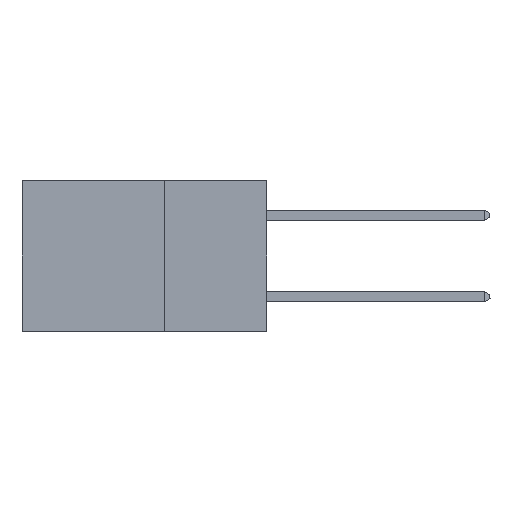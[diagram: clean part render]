
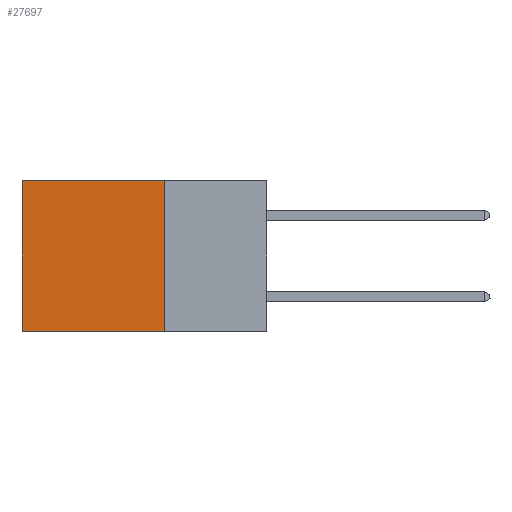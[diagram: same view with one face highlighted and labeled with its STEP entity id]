
A CAD part, left-side view. The second image highlights one B-rep face of the part: STEP entity #27697.
In plain terms, the highlighted planar face has unit normal (-1, 0, 0).
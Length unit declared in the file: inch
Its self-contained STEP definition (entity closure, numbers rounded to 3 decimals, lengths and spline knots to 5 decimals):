
#83 = DIRECTION ( 'NONE',  ( 0., 0., -1. ) ) ;
#556 = VERTEX_POINT ( 'NONE', #36611 ) ;
#962 = DIRECTION ( 'NONE',  ( 0., 0., -1. ) ) ;
#2636 = DIRECTION ( 'NONE',  ( 1., 0., 0. ) ) ;
#3707 = DIRECTION ( 'NONE',  ( 0., 1., 0. ) ) ;
#4337 = LINE ( 'NONE', #6323, #38326 ) ;
#4534 = VERTEX_POINT ( 'NONE', #13665 ) ;
#5148 = EDGE_CURVE ( 'NONE', #4534, #9522, #4337, .T. ) ;
#6323 = CARTESIAN_POINT ( 'NONE',  ( 0.2875, 0.25, 0. ) ) ;
#7136 = CARTESIAN_POINT ( 'NONE',  ( 0.2875, 0.25, 0. ) ) ;
#7503 = CARTESIAN_POINT ( 'NONE',  ( 0.2875, 0.6, 0. ) ) ;
#8552 = ORIENTED_EDGE ( 'NONE', *, *, #16497, .F. ) ;
#9197 = CARTESIAN_POINT ( 'NONE',  ( 0.2875, 0.25, 0. ) ) ;
#9361 = ORIENTED_EDGE ( 'NONE', *, *, #36929, .F. ) ;
#9522 = VERTEX_POINT ( 'NONE', #7503 ) ;
#9742 = DIRECTION ( 'NONE',  ( 0., 1., 0. ) ) ;
#9985 = CARTESIAN_POINT ( 'NONE',  ( 0.2875, 0.25, -0.37 ) ) ;
#11084 = CARTESIAN_POINT ( 'NONE',  ( 0.2875, 0.6, 0. ) ) ;
#13198 = ORIENTED_EDGE ( 'NONE', *, *, #5148, .T. ) ;
#13665 = CARTESIAN_POINT ( 'NONE',  ( 0.2875, 0.25, 0. ) ) ;
#15048 = EDGE_CURVE ( 'NONE', #9522, #26298, #37705, .T. ) ;
#16497 = EDGE_CURVE ( 'NONE', #556, #26298, #33388, .T. ) ;
#17237 = EDGE_LOOP ( 'NONE', ( #17474, #8552, #9361, #13198 ) ) ;
#17474 = ORIENTED_EDGE ( 'NONE', *, *, #15048, .T. ) ;
#19897 = CARTESIAN_POINT ( 'NONE',  ( 0.2875, 0.6, -0.37 ) ) ;
#21868 = PLANE ( 'NONE',  #28758 ) ;
#24857 = FACE_OUTER_BOUND ( 'NONE', #17237, .T. ) ;
#25031 = DIRECTION ( 'NONE',  ( 0., 0., -1. ) ) ;
#25237 = VECTOR ( 'NONE', #962, 39.37008 ) ;
#26298 = VERTEX_POINT ( 'NONE', #19897 ) ;
#27697 = ADVANCED_FACE ( 'NONE', ( #24857 ), #21868, .F. ) ;
#28758 = AXIS2_PLACEMENT_3D ( 'NONE', #9197, #2636, #25031 ) ;
#31104 = LINE ( 'NONE', #7136, #25237 ) ;
#31949 = VECTOR ( 'NONE', #3707, 39.37008 ) ;
#33388 = LINE ( 'NONE', #9985, #31949 ) ;
#36611 = CARTESIAN_POINT ( 'NONE',  ( 0.2875, 0.25, -0.37 ) ) ;
#36929 = EDGE_CURVE ( 'NONE', #4534, #556, #31104, .T. ) ;
#37705 = LINE ( 'NONE', #11084, #38714 ) ;
#38326 = VECTOR ( 'NONE', #9742, 39.37008 ) ;
#38714 = VECTOR ( 'NONE', #83, 39.37008 ) ;
